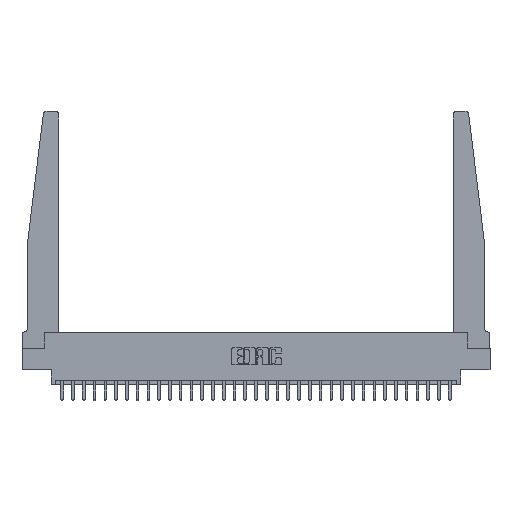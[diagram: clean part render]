
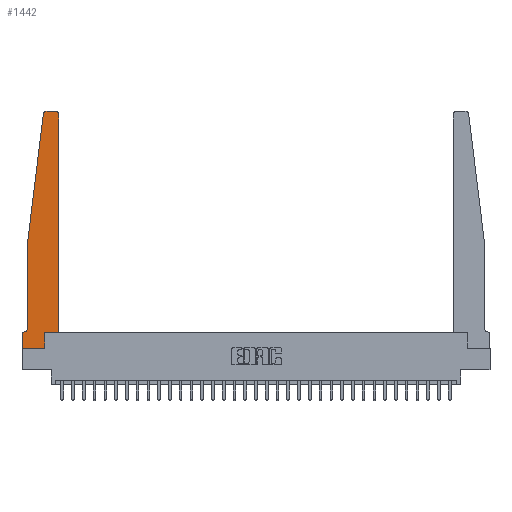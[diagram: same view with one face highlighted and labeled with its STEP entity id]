
A CAD part, top view. The second image highlights one B-rep face of the part: STEP entity #1442.
In plain terms, the highlighted planar face has unit normal (0, 0, 1).
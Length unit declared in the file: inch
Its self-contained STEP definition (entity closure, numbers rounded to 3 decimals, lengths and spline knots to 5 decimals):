
#987 = CARTESIAN_POINT ( 'NONE',  ( 0., 0., 0.37 ) ) ;
#1079 = LINE ( 'NONE', #22403, #16857 ) ;
#1401 = DIRECTION ( 'NONE',  ( 1., 0., 0. ) ) ;
#1424 = DIRECTION ( 'NONE',  ( -0.122, -0.992, 0. ) ) ;
#1442 = ADVANCED_FACE ( 'NONE', ( #17659 ), #22111, .T. ) ;
#1826 = ORIENTED_EDGE ( 'NONE', *, *, #8709, .T. ) ;
#2053 = AXIS2_PLACEMENT_3D ( 'NONE', #23765, #26222, #11788 ) ;
#2818 = ORIENTED_EDGE ( 'NONE', *, *, #7189, .T. ) ;
#3023 = CARTESIAN_POINT ( 'NONE',  ( 0.395, 2.72, 0.37 ) ) ;
#3189 = VERTEX_POINT ( 'NONE', #17629 ) ;
#3632 = DIRECTION ( 'NONE',  ( 0., 1., 0. ) ) ;
#3898 = EDGE_CURVE ( 'NONE', #8489, #16383, #7333, .T. ) ;
#5494 = LINE ( 'NONE', #15261, #20311 ) ;
#5554 = LINE ( 'NONE', #10621, #29205 ) ;
#5808 = EDGE_CURVE ( 'NONE', #28486, #8212, #26930, .T. ) ;
#6418 = DIRECTION ( 'NONE',  ( 1., 0., 0. ) ) ;
#6473 = CARTESIAN_POINT ( 'NONE',  ( 0.065, 0.1875, 0.37 ) ) ;
#6834 = CARTESIAN_POINT ( 'NONE',  ( 0.425, 0.18, 0.37 ) ) ;
#7189 = EDGE_CURVE ( 'NONE', #20082, #28410, #5494, .T. ) ;
#7333 = LINE ( 'NONE', #7649, #23491 ) ;
#7407 = CARTESIAN_POINT ( 'NONE',  ( 0.425, 0.18, 0.37 ) ) ;
#7649 = CARTESIAN_POINT ( 'NONE',  ( 0., 0., 0.37 ) ) ;
#7764 = VERTEX_POINT ( 'NONE', #21514 ) ;
#7926 = DIRECTION ( 'NONE',  ( 1., 0., 0. ) ) ;
#7966 = VECTOR ( 'NONE', #18672, 39.37008 ) ;
#8192 = LINE ( 'NONE', #987, #15837 ) ;
#8212 = VERTEX_POINT ( 'NONE', #18866 ) ;
#8489 = VERTEX_POINT ( 'NONE', #22239 ) ;
#8585 = CIRCLE ( 'NONE', #12499, 0.03 ) ;
#8709 = EDGE_CURVE ( 'NONE', #7764, #26443, #28181, .T. ) ;
#8777 = LINE ( 'NONE', #6473, #21207 ) ;
#9307 = CARTESIAN_POINT ( 'NONE',  ( 0.065, 0.2375, 0.37 ) ) ;
#9974 = ORIENTED_EDGE ( 'NONE', *, *, #3898, .T. ) ;
#10223 = CARTESIAN_POINT ( 'NONE',  ( 0.25, 2.75, 0.37 ) ) ;
#10342 = DIRECTION ( 'NONE',  ( 1., 0., 0. ) ) ;
#10456 = ORIENTED_EDGE ( 'NONE', *, *, #5808, .T. ) ;
#10621 = CARTESIAN_POINT ( 'NONE',  ( 0.065, 1.25, 0.37 ) ) ;
#11506 = EDGE_CURVE ( 'NONE', #26443, #28486, #13827, .T. ) ;
#11623 = LINE ( 'NONE', #6834, #16834 ) ;
#11634 = DIRECTION ( 'NONE',  ( 0., -1., 0. ) ) ;
#11788 = DIRECTION ( 'NONE',  ( -1., 0., 0. ) ) ;
#12499 = AXIS2_PLACEMENT_3D ( 'NONE', #22626, #27227, #21765 ) ;
#12827 = EDGE_CURVE ( 'NONE', #21350, #20565, #1079, .T. ) ;
#13208 = CARTESIAN_POINT ( 'NONE',  ( 0., 0., 0.37 ) ) ;
#13748 = EDGE_CURVE ( 'NONE', #28077, #8489, #8777, .T. ) ;
#13827 = CIRCLE ( 'NONE', #24628, 0.03 ) ;
#14077 = CARTESIAN_POINT ( 'NONE',  ( 0.065, 1.25, 0.37 ) ) ;
#14903 = CARTESIAN_POINT ( 'NONE',  ( 0.015, 0.1875, 0.37 ) ) ;
#15212 = DIRECTION ( 'NONE',  ( -1., 0., 0. ) ) ;
#15254 = DIRECTION ( 'NONE',  ( -1., 0., 0. ) ) ;
#15261 = CARTESIAN_POINT ( 'NONE',  ( 0.2605, 0.18, 0.37 ) ) ;
#15443 = CARTESIAN_POINT ( 'NONE',  ( 0.395, 2.75, 0.37 ) ) ;
#15837 = VECTOR ( 'NONE', #10342, 39.37008 ) ;
#16383 = VERTEX_POINT ( 'NONE', #13208 ) ;
#16512 = ORIENTED_EDGE ( 'NONE', *, *, #25416, .T. ) ;
#16834 = VECTOR ( 'NONE', #6418, 39.37008 ) ;
#16857 = VECTOR ( 'NONE', #17497, 39.37008 ) ;
#16972 = EDGE_CURVE ( 'NONE', #8212, #3189, #8585, .T. ) ;
#17497 = DIRECTION ( 'NONE',  ( 0., -1., 0. ) ) ;
#17513 = CARTESIAN_POINT ( 'NONE',  ( 0., 0.1875, 0.37 ) ) ;
#17617 = EDGE_LOOP ( 'NONE', ( #10456, #23720, #24829, #29283, #28075, #28683, #9974, #22611, #2818, #16512, #1826, #26171 ) ) ;
#17629 = CARTESIAN_POINT ( 'NONE',  ( 0.24675, 2.72367, 0.37 ) ) ;
#17659 = FACE_OUTER_BOUND ( 'NONE', #17617, .T. ) ;
#18672 = DIRECTION ( 'NONE',  ( 0., 1., 0. ) ) ;
#18866 = CARTESIAN_POINT ( 'NONE',  ( 0.27653, 2.75, 0.37 ) ) ;
#20082 = VERTEX_POINT ( 'NONE', #29442 ) ;
#20311 = VECTOR ( 'NONE', #3632, 39.37008 ) ;
#20565 = VERTEX_POINT ( 'NONE', #9307 ) ;
#21207 = VECTOR ( 'NONE', #15212, 39.37008 ) ;
#21283 = DIRECTION ( 'NONE',  ( 0., 0., 1. ) ) ;
#21350 = VERTEX_POINT ( 'NONE', #14077 ) ;
#21362 = EDGE_CURVE ( 'NONE', #20565, #28077, #28482, .T. ) ;
#21514 = CARTESIAN_POINT ( 'NONE',  ( 0.425, 0.18, 0.37 ) ) ;
#21765 = DIRECTION ( 'NONE',  ( 1., 0., 0. ) ) ;
#22111 = PLANE ( 'NONE',  #25419 ) ;
#22239 = CARTESIAN_POINT ( 'NONE',  ( 0., 0.1875, 0.37 ) ) ;
#22403 = CARTESIAN_POINT ( 'NONE',  ( 0.065, 1.25, 0.37 ) ) ;
#22611 = ORIENTED_EDGE ( 'NONE', *, *, #23602, .T. ) ;
#22626 = CARTESIAN_POINT ( 'NONE',  ( 0.27653, 2.72, 0.37 ) ) ;
#23491 = VECTOR ( 'NONE', #11634, 39.37008 ) ;
#23602 = EDGE_CURVE ( 'NONE', #16383, #20082, #8192, .T. ) ;
#23720 = ORIENTED_EDGE ( 'NONE', *, *, #16972, .T. ) ;
#23765 = CARTESIAN_POINT ( 'NONE',  ( 0.015, 0.2375, 0.37 ) ) ;
#24628 = AXIS2_PLACEMENT_3D ( 'NONE', #3023, #21283, #7926 ) ;
#24717 = DIRECTION ( 'NONE',  ( 0., 0., 1. ) ) ;
#24829 = ORIENTED_EDGE ( 'NONE', *, *, #28140, .T. ) ;
#25416 = EDGE_CURVE ( 'NONE', #28410, #7764, #11623, .T. ) ;
#25419 = AXIS2_PLACEMENT_3D ( 'NONE', #17513, #24717, #1401 ) ;
#25934 = CARTESIAN_POINT ( 'NONE',  ( 0.2605, 0.18, 0.37 ) ) ;
#26171 = ORIENTED_EDGE ( 'NONE', *, *, #11506, .T. ) ;
#26222 = DIRECTION ( 'NONE',  ( 0., 0., -1. ) ) ;
#26443 = VERTEX_POINT ( 'NONE', #27297 ) ;
#26930 = LINE ( 'NONE', #10223, #27990 ) ;
#27227 = DIRECTION ( 'NONE',  ( 0., 0., 1. ) ) ;
#27297 = CARTESIAN_POINT ( 'NONE',  ( 0.425, 2.72, 0.37 ) ) ;
#27990 = VECTOR ( 'NONE', #15254, 39.37008 ) ;
#28075 = ORIENTED_EDGE ( 'NONE', *, *, #21362, .T. ) ;
#28077 = VERTEX_POINT ( 'NONE', #14903 ) ;
#28140 = EDGE_CURVE ( 'NONE', #3189, #21350, #5554, .T. ) ;
#28181 = LINE ( 'NONE', #7407, #7966 ) ;
#28410 = VERTEX_POINT ( 'NONE', #25934 ) ;
#28482 = CIRCLE ( 'NONE', #2053, 0.05 ) ;
#28486 = VERTEX_POINT ( 'NONE', #15443 ) ;
#28683 = ORIENTED_EDGE ( 'NONE', *, *, #13748, .T. ) ;
#29205 = VECTOR ( 'NONE', #1424, 39.37008 ) ;
#29283 = ORIENTED_EDGE ( 'NONE', *, *, #12827, .T. ) ;
#29442 = CARTESIAN_POINT ( 'NONE',  ( 0.2605, 0., 0.37 ) ) ;
